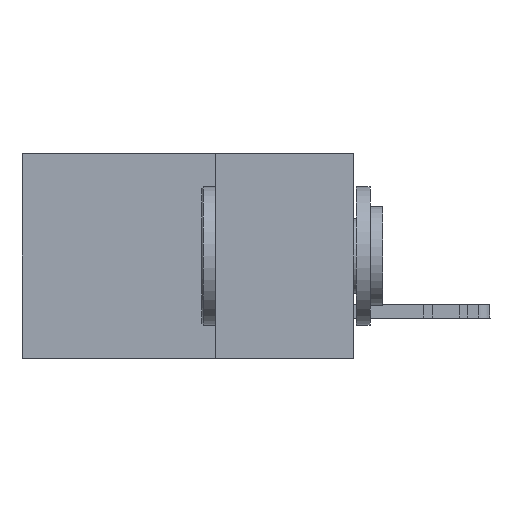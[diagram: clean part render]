
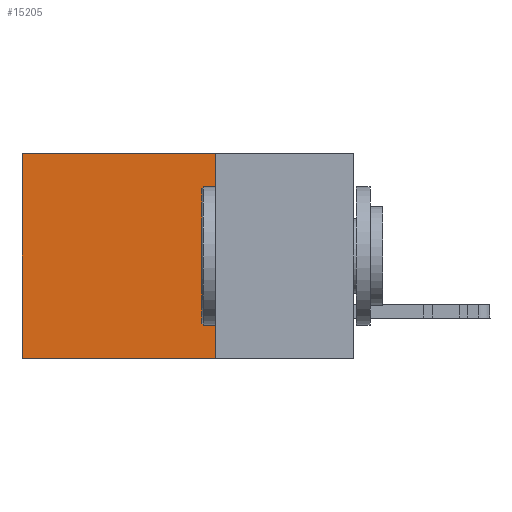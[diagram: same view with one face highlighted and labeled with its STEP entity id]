
A CAD part, left-side view. The second image highlights one B-rep face of the part: STEP entity #15205.
In plain terms, the highlighted planar face has unit normal (-1, 0, 0).
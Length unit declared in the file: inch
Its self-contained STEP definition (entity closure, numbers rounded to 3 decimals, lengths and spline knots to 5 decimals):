
#1134 = VERTEX_POINT ( 'NONE', #11698 ) ;
#2091 = DIRECTION ( 'NONE',  ( 1., 0., 0. ) ) ;
#2875 = ORIENTED_EDGE ( 'NONE', *, *, #12356, .T. ) ;
#4291 = CARTESIAN_POINT ( 'NONE',  ( 0.2875, 0.25, 0. ) ) ;
#4681 = CARTESIAN_POINT ( 'NONE',  ( 0.2875, 0.25, 0. ) ) ;
#6580 = CARTESIAN_POINT ( 'NONE',  ( 0.2875, 0.25, 0. ) ) ;
#6844 = CARTESIAN_POINT ( 'NONE',  ( 0.2875, 0.6, 0. ) ) ;
#9172 = EDGE_CURVE ( 'NONE', #37541, #16211, #24166, .T. ) ;
#9492 = DIRECTION ( 'NONE',  ( 0., 1., 0. ) ) ;
#11633 = VERTEX_POINT ( 'NONE', #6580 ) ;
#11698 = CARTESIAN_POINT ( 'NONE',  ( 0.2875, 0.25, -0.37 ) ) ;
#11817 = CARTESIAN_POINT ( 'NONE',  ( 0.2875, 0.6, 0. ) ) ;
#12261 = LINE ( 'NONE', #41618, #15824 ) ;
#12356 = EDGE_CURVE ( 'NONE', #11633, #37541, #12261, .T. ) ;
#12749 = VECTOR ( 'NONE', #27390, 39.37008 ) ;
#13247 = EDGE_CURVE ( 'NONE', #11633, #1134, #20030, .T. ) ;
#15205 = ADVANCED_FACE ( 'NONE', ( #31485 ), #30665, .F. ) ;
#15824 = VECTOR ( 'NONE', #24816, 39.37008 ) ;
#16211 = VERTEX_POINT ( 'NONE', #32792 ) ;
#19209 = VECTOR ( 'NONE', #9492, 39.37008 ) ;
#19544 = ORIENTED_EDGE ( 'NONE', *, *, #9172, .T. ) ;
#20030 = LINE ( 'NONE', #4291, #23236 ) ;
#23236 = VECTOR ( 'NONE', #23677, 39.37008 ) ;
#23677 = DIRECTION ( 'NONE',  ( 0., 0., -1. ) ) ;
#24166 = LINE ( 'NONE', #11817, #12749 ) ;
#24816 = DIRECTION ( 'NONE',  ( 0., 1., 0. ) ) ;
#25886 = CARTESIAN_POINT ( 'NONE',  ( 0.2875, 0.25, -0.37 ) ) ;
#27390 = DIRECTION ( 'NONE',  ( 0., 0., -1. ) ) ;
#27429 = AXIS2_PLACEMENT_3D ( 'NONE', #4681, #2091, #37666 ) ;
#28277 = EDGE_LOOP ( 'NONE', ( #19544, #29186, #39609, #2875 ) ) ;
#29186 = ORIENTED_EDGE ( 'NONE', *, *, #30757, .F. ) ;
#30665 = PLANE ( 'NONE',  #27429 ) ;
#30757 = EDGE_CURVE ( 'NONE', #1134, #16211, #38649, .T. ) ;
#31485 = FACE_OUTER_BOUND ( 'NONE', #28277, .T. ) ;
#32792 = CARTESIAN_POINT ( 'NONE',  ( 0.2875, 0.6, -0.37 ) ) ;
#37541 = VERTEX_POINT ( 'NONE', #6844 ) ;
#37666 = DIRECTION ( 'NONE',  ( 0., 0., -1. ) ) ;
#38649 = LINE ( 'NONE', #25886, #19209 ) ;
#39609 = ORIENTED_EDGE ( 'NONE', *, *, #13247, .F. ) ;
#41618 = CARTESIAN_POINT ( 'NONE',  ( 0.2875, 0.25, 0. ) ) ;
